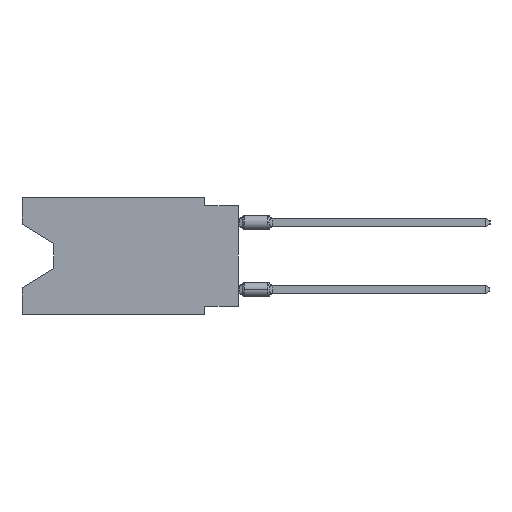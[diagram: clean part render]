
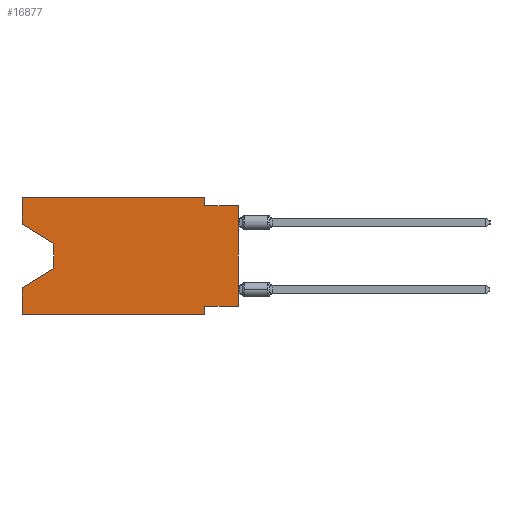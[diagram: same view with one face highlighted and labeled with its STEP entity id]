
A CAD part, left-side view. The second image highlights one B-rep face of the part: STEP entity #16877.
In plain terms, the highlighted planar face has unit normal (-1, 0, 0).
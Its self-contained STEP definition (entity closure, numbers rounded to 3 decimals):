
#296 = LINE ( 'NONE', #28583, #14125 ) ;
#778 = LINE ( 'NONE', #11276, #25570 ) ;
#1252 = VECTOR ( 'NONE', #58133, 1000. ) ;
#1381 = LINE ( 'NONE', #24836, #14049 ) ;
#1454 = VERTEX_POINT ( 'NONE', #14505 ) ;
#1875 = LINE ( 'NONE', #47587, #7160 ) ;
#1981 = VERTEX_POINT ( 'NONE', #51107 ) ;
#2064 = VERTEX_POINT ( 'NONE', #35433 ) ;
#3113 = DIRECTION ( 'NONE',  ( 0., -1., 0. ) ) ;
#4169 = EDGE_CURVE ( 'NONE', #17286, #47762, #25683, .T. ) ;
#4396 = CARTESIAN_POINT ( 'NONE',  ( 0., 16.383, 0. ) ) ;
#5274 = VERTEX_POINT ( 'NONE', #35501 ) ;
#6254 = VECTOR ( 'NONE', #51237, 1000. ) ;
#6797 = ORIENTED_EDGE ( 'NONE', *, *, #11260, .T. ) ;
#7160 = VECTOR ( 'NONE', #25032, 1000. ) ;
#7952 = ORIENTED_EDGE ( 'NONE', *, *, #31754, .T. ) ;
#8395 = LINE ( 'NONE', #21936, #25809 ) ;
#10189 = CARTESIAN_POINT ( 'NONE',  ( 0., 13.97, -5.385 ) ) ;
#10348 = DIRECTION ( 'NONE',  ( 0., 0., -1. ) ) ;
#10864 = VERTEX_POINT ( 'NONE', #34926 ) ;
#11260 = EDGE_CURVE ( 'NONE', #2064, #5274, #17292, .T. ) ;
#11276 = CARTESIAN_POINT ( 'NONE',  ( 0., 16.383, 0. ) ) ;
#11589 = ORIENTED_EDGE ( 'NONE', *, *, #37075, .F. ) ;
#12615 = FACE_OUTER_BOUND ( 'NONE', #26461, .T. ) ;
#12679 = EDGE_CURVE ( 'NONE', #39834, #20309, #27820, .T. ) ;
#12900 = DIRECTION ( 'NONE',  ( 0., 0., -1. ) ) ;
#14049 = VECTOR ( 'NONE', #52193, 1000. ) ;
#14125 = VECTOR ( 'NONE', #55338, 1000. ) ;
#14336 = EDGE_CURVE ( 'NONE', #1454, #21053, #1381, .T. ) ;
#14505 = CARTESIAN_POINT ( 'NONE',  ( 0., 16.383, -2.038 ) ) ;
#15534 = ORIENTED_EDGE ( 'NONE', *, *, #20899, .F. ) ;
#16076 = LINE ( 'NONE', #25690, #22492 ) ;
#16708 = DIRECTION ( 'NONE',  ( 0., -1., 0. ) ) ;
#16877 = ADVANCED_FACE ( 'NONE', ( #12615 ), #22030, .F. ) ;
#17286 = VERTEX_POINT ( 'NONE', #57288 ) ;
#17292 = LINE ( 'NONE', #54566, #25189 ) ;
#20309 = VERTEX_POINT ( 'NONE', #43177 ) ;
#20899 = EDGE_CURVE ( 'NONE', #10864, #5274, #8395, .T. ) ;
#21053 = VERTEX_POINT ( 'NONE', #38521 ) ;
#21241 = CARTESIAN_POINT ( 'NONE',  ( 0., 0., -8.255 ) ) ;
#21404 = CARTESIAN_POINT ( 'NONE',  ( 0., 2.54, -0.635 ) ) ;
#21620 = EDGE_CURVE ( 'NONE', #21053, #17286, #22452, .T. ) ;
#21936 = CARTESIAN_POINT ( 'NONE',  ( 0., 2.54, -8.89 ) ) ;
#22030 = PLANE ( 'NONE',  #45945 ) ;
#22452 = LINE ( 'NONE', #4396, #36413 ) ;
#22492 = VECTOR ( 'NONE', #3113, 1000. ) ;
#24814 = DIRECTION ( 'NONE',  ( 0., 0., 1. ) ) ;
#24836 = CARTESIAN_POINT ( 'NONE',  ( 0., 16.383, 0. ) ) ;
#25032 = DIRECTION ( 'NONE',  ( 0., 1., 0. ) ) ;
#25189 = VECTOR ( 'NONE', #16708, 1000. ) ;
#25461 = ORIENTED_EDGE ( 'NONE', *, *, #21620, .F. ) ;
#25570 = VECTOR ( 'NONE', #24814, 1000. ) ;
#25683 = LINE ( 'NONE', #39817, #1252 ) ;
#25690 = CARTESIAN_POINT ( 'NONE',  ( 0., 0., -0.635 ) ) ;
#25809 = VECTOR ( 'NONE', #12900, 1000. ) ;
#26454 = CARTESIAN_POINT ( 'NONE',  ( 0., 16.383, 0. ) ) ;
#26461 = EDGE_LOOP ( 'NONE', ( #59406, #56045, #35864, #38982, #6797, #15534, #11589, #7952, #39027, #41457, #25461, #29277 ) ) ;
#27820 = LINE ( 'NONE', #46454, #51239 ) ;
#28122 = CARTESIAN_POINT ( 'NONE',  ( 0., 0., -0.635 ) ) ;
#28583 = CARTESIAN_POINT ( 'NONE',  ( 0., 0., 0. ) ) ;
#29277 = ORIENTED_EDGE ( 'NONE', *, *, #14336, .F. ) ;
#31754 = EDGE_CURVE ( 'NONE', #40849, #54175, #296, .T. ) ;
#32923 = CARTESIAN_POINT ( 'NONE',  ( 0., 13.97, -3.505 ) ) ;
#34865 = EDGE_CURVE ( 'NONE', #47762, #54175, #16076, .T. ) ;
#34926 = CARTESIAN_POINT ( 'NONE',  ( 0., 2.54, -8.255 ) ) ;
#35433 = CARTESIAN_POINT ( 'NONE',  ( 0., 16.383, -8.89 ) ) ;
#35501 = CARTESIAN_POINT ( 'NONE',  ( 0., 2.54, -8.89 ) ) ;
#35864 = ORIENTED_EDGE ( 'NONE', *, *, #55430, .T. ) ;
#36413 = VECTOR ( 'NONE', #59125, 1000. ) ;
#37075 = EDGE_CURVE ( 'NONE', #40849, #10864, #1875, .T. ) ;
#38521 = CARTESIAN_POINT ( 'NONE',  ( 0., 16.383, 0. ) ) ;
#38982 = ORIENTED_EDGE ( 'NONE', *, *, #48333, .F. ) ;
#39027 = ORIENTED_EDGE ( 'NONE', *, *, #34865, .F. ) ;
#39817 = CARTESIAN_POINT ( 'NONE',  ( 0., 2.54, 0. ) ) ;
#39834 = VERTEX_POINT ( 'NONE', #32923 ) ;
#40849 = VERTEX_POINT ( 'NONE', #21241 ) ;
#41202 = DIRECTION ( 'NONE',  ( 1., 0., 0. ) ) ;
#41457 = ORIENTED_EDGE ( 'NONE', *, *, #4169, .F. ) ;
#41943 = CARTESIAN_POINT ( 'NONE',  ( 0., 16.383, -2.038 ) ) ;
#42243 = LINE ( 'NONE', #41943, #6254 ) ;
#43177 = CARTESIAN_POINT ( 'NONE',  ( 0., 13.97, -5.385 ) ) ;
#45945 = AXIS2_PLACEMENT_3D ( 'NONE', #26454, #41202, #58912 ) ;
#46011 = DIRECTION ( 'NONE',  ( 0., 0.855, -0.519 ) ) ;
#46454 = CARTESIAN_POINT ( 'NONE',  ( 0., 13.97, -3.505 ) ) ;
#47587 = CARTESIAN_POINT ( 'NONE',  ( 0., 0., -8.255 ) ) ;
#47762 = VERTEX_POINT ( 'NONE', #21404 ) ;
#48333 = EDGE_CURVE ( 'NONE', #2064, #1981, #778, .T. ) ;
#51107 = CARTESIAN_POINT ( 'NONE',  ( 0., 16.383, -6.852 ) ) ;
#51237 = DIRECTION ( 'NONE',  ( 0., -0.855, -0.519 ) ) ;
#51239 = VECTOR ( 'NONE', #10348, 1000. ) ;
#51993 = VECTOR ( 'NONE', #46011, 1000. ) ;
#52193 = DIRECTION ( 'NONE',  ( 0., 0., 1. ) ) ;
#54175 = VERTEX_POINT ( 'NONE', #28122 ) ;
#54566 = CARTESIAN_POINT ( 'NONE',  ( 0., 16.383, -8.89 ) ) ;
#55338 = DIRECTION ( 'NONE',  ( 0., 0., 1. ) ) ;
#55430 = EDGE_CURVE ( 'NONE', #20309, #1981, #55909, .T. ) ;
#55909 = LINE ( 'NONE', #10189, #51993 ) ;
#56045 = ORIENTED_EDGE ( 'NONE', *, *, #12679, .T. ) ;
#57288 = CARTESIAN_POINT ( 'NONE',  ( 0., 2.54, 0. ) ) ;
#58133 = DIRECTION ( 'NONE',  ( 0., 0., -1. ) ) ;
#58481 = EDGE_CURVE ( 'NONE', #1454, #39834, #42243, .T. ) ;
#58912 = DIRECTION ( 'NONE',  ( 0., 0., -1. ) ) ;
#59125 = DIRECTION ( 'NONE',  ( 0., -1., 0. ) ) ;
#59406 = ORIENTED_EDGE ( 'NONE', *, *, #58481, .T. ) ;
